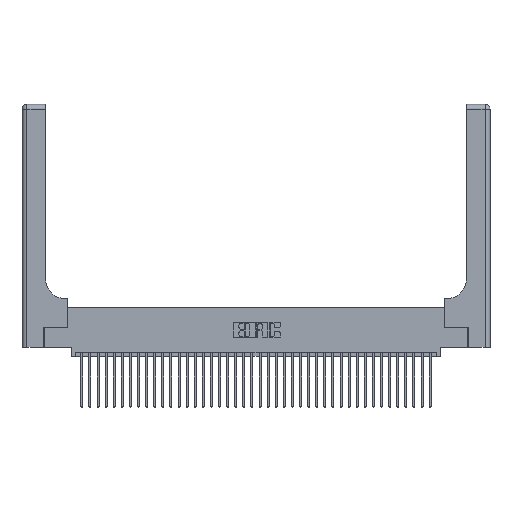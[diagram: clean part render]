
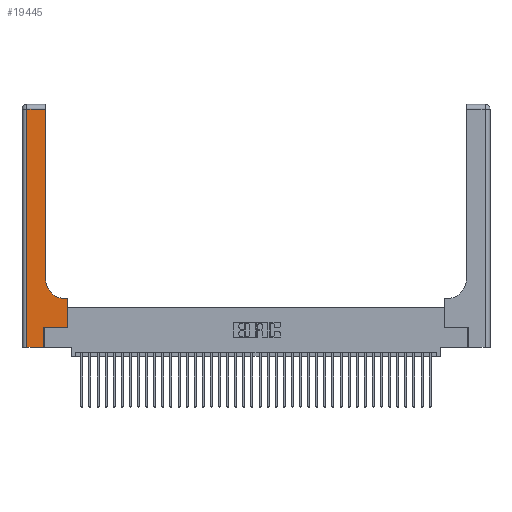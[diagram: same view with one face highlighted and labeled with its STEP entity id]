
A CAD part, top view. The second image highlights one B-rep face of the part: STEP entity #19445.
In plain terms, the highlighted planar face has unit normal (0, 0, 1).
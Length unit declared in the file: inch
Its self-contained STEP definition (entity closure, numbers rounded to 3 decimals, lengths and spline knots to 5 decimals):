
#111 = VECTOR ( 'NONE', #28727, 39.37008 ) ;
#2048 = DIRECTION ( 'NONE',  ( 0., 1., 0. ) ) ;
#2212 = CARTESIAN_POINT ( 'NONE',  ( 0.269, 0., 0.37 ) ) ;
#2449 = DIRECTION ( 'NONE',  ( 1., 0., 0. ) ) ;
#3917 = EDGE_CURVE ( 'NONE', #37061, #29380, #31676, .T. ) ;
#3958 = LINE ( 'NONE', #35163, #111 ) ;
#4704 = ORIENTED_EDGE ( 'NONE', *, *, #18452, .T. ) ;
#4922 = LINE ( 'NONE', #35728, #25025 ) ;
#5671 = VECTOR ( 'NONE', #28444, 39.37008 ) ;
#6818 = ORIENTED_EDGE ( 'NONE', *, *, #13480, .T. ) ;
#8001 = CARTESIAN_POINT ( 'NONE',  ( 0.06, 0., 0.37 ) ) ;
#8564 = ORIENTED_EDGE ( 'NONE', *, *, #16792, .T. ) ;
#10037 = VECTOR ( 'NONE', #24592, 39.37008 ) ;
#10213 = VECTOR ( 'NONE', #19650, 39.37008 ) ;
#11173 = DIRECTION ( 'NONE',  ( 0., 1., 0. ) ) ;
#11378 = FACE_OUTER_BOUND ( 'NONE', #21466, .T. ) ;
#11583 = CARTESIAN_POINT ( 'NONE',  ( 0.5585, 0.6, 0.37 ) ) ;
#12168 = CARTESIAN_POINT ( 'NONE',  ( 0.2915, 0.6, 0.37 ) ) ;
#12216 = VECTOR ( 'NONE', #2048, 39.37008 ) ;
#13480 = EDGE_CURVE ( 'NONE', #33373, #39560, #33958, .T. ) ;
#13679 = VERTEX_POINT ( 'NONE', #11583 ) ;
#13692 = AXIS2_PLACEMENT_3D ( 'NONE', #35824, #23796, #35567 ) ;
#13825 = CARTESIAN_POINT ( 'NONE',  ( 0., 3., 0.37 ) ) ;
#13958 = DIRECTION ( 'NONE',  ( -1., 0., 0. ) ) ;
#14011 = LINE ( 'NONE', #16444, #10213 ) ;
#15931 = CARTESIAN_POINT ( 'NONE',  ( 0.2915, 0.85, 0.37 ) ) ;
#16126 = EDGE_CURVE ( 'NONE', #29380, #21546, #4922, .T. ) ;
#16128 = VERTEX_POINT ( 'NONE', #20625 ) ;
#16299 = EDGE_CURVE ( 'NONE', #29970, #13679, #14011, .T. ) ;
#16444 = CARTESIAN_POINT ( 'NONE',  ( 0.5585, 0.25, 0.37 ) ) ;
#16792 = EDGE_CURVE ( 'NONE', #39560, #37061, #3958, .T. ) ;
#18452 = EDGE_CURVE ( 'NONE', #13679, #16128, #36785, .T. ) ;
#19119 = CARTESIAN_POINT ( 'NONE',  ( 0.06, 3., 0.37 ) ) ;
#19122 = EDGE_CURVE ( 'NONE', #22771, #29970, #31970, .T. ) ;
#19206 = CARTESIAN_POINT ( 'NONE',  ( 0.269, 0.25, 0.37 ) ) ;
#19369 = DIRECTION ( 'NONE',  ( 0., -1., 0. ) ) ;
#19445 = ADVANCED_FACE ( 'NONE', ( #11378 ), #23185, .F. ) ;
#19650 = DIRECTION ( 'NONE',  ( 0., 1., 0. ) ) ;
#19671 = ORIENTED_EDGE ( 'NONE', *, *, #19122, .T. ) ;
#20380 = DIRECTION ( 'NONE',  ( 0., 0., -1. ) ) ;
#20393 = ORIENTED_EDGE ( 'NONE', *, *, #16299, .T. ) ;
#20480 = AXIS2_PLACEMENT_3D ( 'NONE', #13825, #20380, #13958 ) ;
#20625 = CARTESIAN_POINT ( 'NONE',  ( 0.5415, 0.6, 0.37 ) ) ;
#21466 = EDGE_LOOP ( 'NONE', ( #6818, #8564, #31998, #24153, #23008, #19671, #20393, #4704, #29615 ) ) ;
#21546 = VERTEX_POINT ( 'NONE', #2212 ) ;
#22600 = CIRCLE ( 'NONE', #13692, 0.25 ) ;
#22771 = VERTEX_POINT ( 'NONE', #33672 ) ;
#22899 = VECTOR ( 'NONE', #11173, 39.37008 ) ;
#23008 = ORIENTED_EDGE ( 'NONE', *, *, #30052, .T. ) ;
#23185 = PLANE ( 'NONE',  #20480 ) ;
#23796 = DIRECTION ( 'NONE',  ( 0., 0., -1. ) ) ;
#24153 = ORIENTED_EDGE ( 'NONE', *, *, #16126, .T. ) ;
#24592 = DIRECTION ( 'NONE',  ( -1., 0., 0. ) ) ;
#25025 = VECTOR ( 'NONE', #2449, 39.37008 ) ;
#25318 = CARTESIAN_POINT ( 'NONE',  ( 0.5585, 0.25, 0.37 ) ) ;
#26093 = CARTESIAN_POINT ( 'NONE',  ( 0.269, 0., 0.37 ) ) ;
#28444 = DIRECTION ( 'NONE',  ( 1., 0., 0. ) ) ;
#28527 = LINE ( 'NONE', #26093, #12216 ) ;
#28727 = DIRECTION ( 'NONE',  ( -1., 0., 0. ) ) ;
#29380 = VERTEX_POINT ( 'NONE', #8001 ) ;
#29615 = ORIENTED_EDGE ( 'NONE', *, *, #36751, .T. ) ;
#29970 = VERTEX_POINT ( 'NONE', #25318 ) ;
#30052 = EDGE_CURVE ( 'NONE', #21546, #22771, #28527, .T. ) ;
#31676 = LINE ( 'NONE', #19119, #32115 ) ;
#31970 = LINE ( 'NONE', #19206, #5671 ) ;
#31998 = ORIENTED_EDGE ( 'NONE', *, *, #3917, .T. ) ;
#32115 = VECTOR ( 'NONE', #19369, 39.37008 ) ;
#33134 = CARTESIAN_POINT ( 'NONE',  ( 0.2915, 2.94, 0.37 ) ) ;
#33373 = VERTEX_POINT ( 'NONE', #15931 ) ;
#33672 = CARTESIAN_POINT ( 'NONE',  ( 0.269, 0.25, 0.37 ) ) ;
#33842 = CARTESIAN_POINT ( 'NONE',  ( 0.06, 2.94, 0.37 ) ) ;
#33958 = LINE ( 'NONE', #38187, #22899 ) ;
#35163 = CARTESIAN_POINT ( 'NONE',  ( 0., 2.94, 0.37 ) ) ;
#35567 = DIRECTION ( 'NONE',  ( 1., 0., 0. ) ) ;
#35728 = CARTESIAN_POINT ( 'NONE',  ( 0., 0., 0.37 ) ) ;
#35824 = CARTESIAN_POINT ( 'NONE',  ( 0.5415, 0.85, 0.37 ) ) ;
#36751 = EDGE_CURVE ( 'NONE', #16128, #33373, #22600, .T. ) ;
#36785 = LINE ( 'NONE', #12168, #10037 ) ;
#37061 = VERTEX_POINT ( 'NONE', #33842 ) ;
#38187 = CARTESIAN_POINT ( 'NONE',  ( 0.2915, 3., 0.37 ) ) ;
#39560 = VERTEX_POINT ( 'NONE', #33134 ) ;
